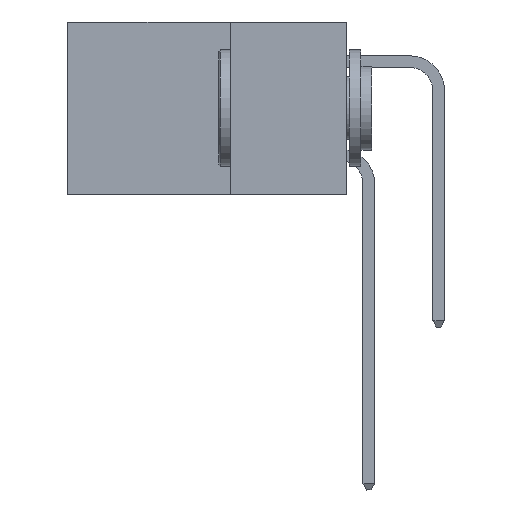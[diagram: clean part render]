
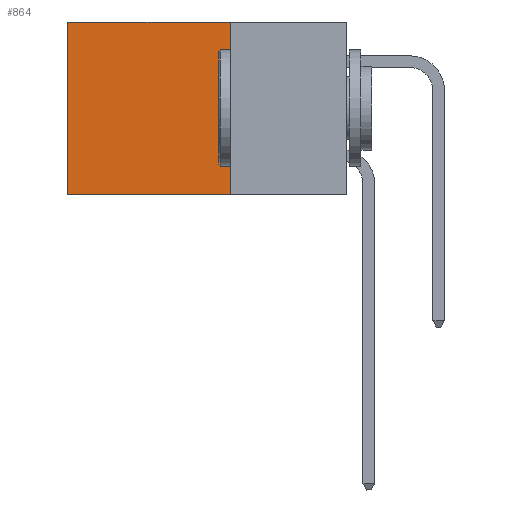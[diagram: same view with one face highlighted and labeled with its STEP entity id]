
A CAD part, left-side view. The second image highlights one B-rep face of the part: STEP entity #864.
In plain terms, the highlighted planar face has unit normal (-1, 0, 0).
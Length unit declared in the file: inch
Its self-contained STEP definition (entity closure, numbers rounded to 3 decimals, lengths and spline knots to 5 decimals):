
#50 = EDGE_CURVE ( 'NONE', #9068, #4987, #545, .T. ) ;
#238 = EDGE_CURVE ( 'NONE', #17548, #27161, #28635, .T. ) ;
#545 = LINE ( 'NONE', #8547, #27943 ) ;
#715 = CARTESIAN_POINT ( 'NONE',  ( 0.2875, 0.25, 0. ) ) ;
#864 = ADVANCED_FACE ( 'NONE', ( #24702 ), #7277, .F. ) ;
#2754 = LINE ( 'NONE', #15717, #11272 ) ;
#4987 = VERTEX_POINT ( 'NONE', #19029 ) ;
#6217 = ORIENTED_EDGE ( 'NONE', *, *, #6292, .T. ) ;
#6292 = EDGE_CURVE ( 'NONE', #9068, #17548, #2754, .T. ) ;
#7277 = PLANE ( 'NONE',  #19426 ) ;
#7918 = EDGE_CURVE ( 'NONE', #4987, #27161, #24364, .T. ) ;
#8166 = DIRECTION ( 'NONE',  ( 0., 1., 0. ) ) ;
#8547 = CARTESIAN_POINT ( 'NONE',  ( 0.2875, 0.25, 0. ) ) ;
#9068 = VERTEX_POINT ( 'NONE', #14500 ) ;
#9597 = ORIENTED_EDGE ( 'NONE', *, *, #50, .F. ) ;
#10470 = VECTOR ( 'NONE', #8166, 39.37008 ) ;
#11272 = VECTOR ( 'NONE', #22702, 39.37008 ) ;
#11573 = VECTOR ( 'NONE', #27708, 39.37008 ) ;
#12164 = DIRECTION ( 'NONE',  ( 0., 0., -1. ) ) ;
#12646 = CARTESIAN_POINT ( 'NONE',  ( 0.2875, 0.25, -0.37 ) ) ;
#14500 = CARTESIAN_POINT ( 'NONE',  ( 0.2875, 0.25, 0. ) ) ;
#14554 = ORIENTED_EDGE ( 'NONE', *, *, #7918, .F. ) ;
#15717 = CARTESIAN_POINT ( 'NONE',  ( 0.2875, 0.25, 0. ) ) ;
#17548 = VERTEX_POINT ( 'NONE', #27281 ) ;
#18104 = CARTESIAN_POINT ( 'NONE',  ( 0.2875, 0.6, 0. ) ) ;
#19029 = CARTESIAN_POINT ( 'NONE',  ( 0.2875, 0.25, -0.37 ) ) ;
#19426 = AXIS2_PLACEMENT_3D ( 'NONE', #715, #27775, #12164 ) ;
#22702 = DIRECTION ( 'NONE',  ( 0., 1., 0. ) ) ;
#23766 = DIRECTION ( 'NONE',  ( 0., 0., -1. ) ) ;
#24364 = LINE ( 'NONE', #12646, #10470 ) ;
#24702 = FACE_OUTER_BOUND ( 'NONE', #27276, .T. ) ;
#26150 = ORIENTED_EDGE ( 'NONE', *, *, #238, .T. ) ;
#27161 = VERTEX_POINT ( 'NONE', #27630 ) ;
#27276 = EDGE_LOOP ( 'NONE', ( #26150, #14554, #9597, #6217 ) ) ;
#27281 = CARTESIAN_POINT ( 'NONE',  ( 0.2875, 0.6, 0. ) ) ;
#27630 = CARTESIAN_POINT ( 'NONE',  ( 0.2875, 0.6, -0.37 ) ) ;
#27708 = DIRECTION ( 'NONE',  ( 0., 0., -1. ) ) ;
#27775 = DIRECTION ( 'NONE',  ( 1., 0., 0. ) ) ;
#27943 = VECTOR ( 'NONE', #23766, 39.37008 ) ;
#28635 = LINE ( 'NONE', #18104, #11573 ) ;
